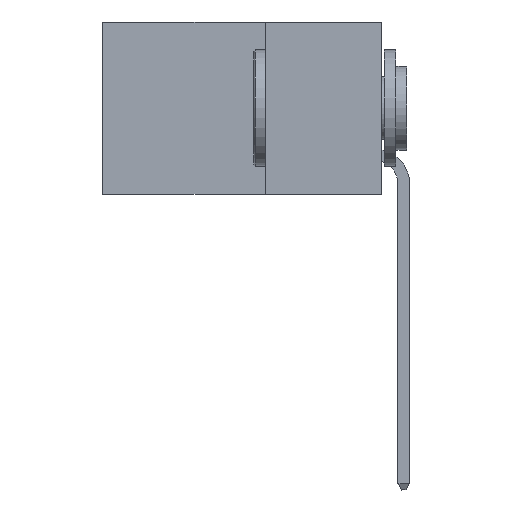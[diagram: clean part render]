
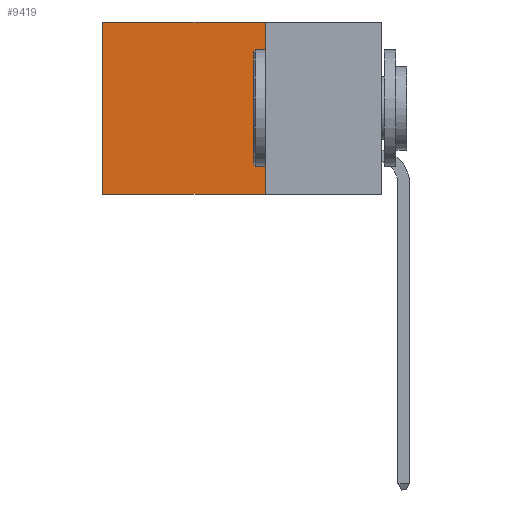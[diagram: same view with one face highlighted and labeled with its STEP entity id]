
A CAD part, left-side view. The second image highlights one B-rep face of the part: STEP entity #9419.
In plain terms, the highlighted planar face has unit normal (-1, 0, 0).
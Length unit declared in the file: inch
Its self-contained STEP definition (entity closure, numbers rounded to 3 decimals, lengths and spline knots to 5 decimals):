
#2 = EDGE_CURVE ( 'NONE', #17617, #24704, #14192, .T. ) ;
#827 = CARTESIAN_POINT ( 'NONE',  ( 0.2875, 0.25, -0.37 ) ) ;
#1540 = LINE ( 'NONE', #19312, #7014 ) ;
#1626 = DIRECTION ( 'NONE',  ( 0., 0., -1. ) ) ;
#1886 = CARTESIAN_POINT ( 'NONE',  ( 0.2875, 0.25, 0. ) ) ;
#3583 = DIRECTION ( 'NONE',  ( 0., 1., 0. ) ) ;
#4084 = DIRECTION ( 'NONE',  ( 0., 0., -1. ) ) ;
#4148 = ORIENTED_EDGE ( 'NONE', *, *, #23896, .F. ) ;
#5484 = VECTOR ( 'NONE', #1626, 39.37008 ) ;
#6017 = PLANE ( 'NONE',  #13813 ) ;
#6112 = DIRECTION ( 'NONE',  ( 0., 0., -1. ) ) ;
#6855 = VERTEX_POINT ( 'NONE', #827 ) ;
#6882 = EDGE_CURVE ( 'NONE', #24704, #18723, #8126, .T. ) ;
#7014 = VECTOR ( 'NONE', #3583, 39.37008 ) ;
#7795 = ORIENTED_EDGE ( 'NONE', *, *, #6882, .T. ) ;
#8126 = LINE ( 'NONE', #9735, #22111 ) ;
#9419 = ADVANCED_FACE ( 'NONE', ( #23034 ), #6017, .F. ) ;
#9735 = CARTESIAN_POINT ( 'NONE',  ( 0.2875, 0.6, 0. ) ) ;
#9984 = CARTESIAN_POINT ( 'NONE',  ( 0.2875, 0.25, 0. ) ) ;
#10827 = CARTESIAN_POINT ( 'NONE',  ( 0.2875, 0.25, 0. ) ) ;
#11217 = DIRECTION ( 'NONE',  ( 0., 1., 0. ) ) ;
#11560 = EDGE_CURVE ( 'NONE', #6855, #18723, #1540, .T. ) ;
#13813 = AXIS2_PLACEMENT_3D ( 'NONE', #10827, #15616, #6112 ) ;
#14192 = LINE ( 'NONE', #1886, #30434 ) ;
#15616 = DIRECTION ( 'NONE',  ( 1., 0., 0. ) ) ;
#17617 = VERTEX_POINT ( 'NONE', #9984 ) ;
#18708 = EDGE_LOOP ( 'NONE', ( #7795, #24937, #4148, #22323 ) ) ;
#18723 = VERTEX_POINT ( 'NONE', #29151 ) ;
#19312 = CARTESIAN_POINT ( 'NONE',  ( 0.2875, 0.25, -0.37 ) ) ;
#22111 = VECTOR ( 'NONE', #4084, 39.37008 ) ;
#22323 = ORIENTED_EDGE ( 'NONE', *, *, #2, .T. ) ;
#22884 = CARTESIAN_POINT ( 'NONE',  ( 0.2875, 0.6, 0. ) ) ;
#23034 = FACE_OUTER_BOUND ( 'NONE', #18708, .T. ) ;
#23178 = LINE ( 'NONE', #27541, #5484 ) ;
#23896 = EDGE_CURVE ( 'NONE', #17617, #6855, #23178, .T. ) ;
#24704 = VERTEX_POINT ( 'NONE', #22884 ) ;
#24937 = ORIENTED_EDGE ( 'NONE', *, *, #11560, .F. ) ;
#27541 = CARTESIAN_POINT ( 'NONE',  ( 0.2875, 0.25, 0. ) ) ;
#29151 = CARTESIAN_POINT ( 'NONE',  ( 0.2875, 0.6, -0.37 ) ) ;
#30434 = VECTOR ( 'NONE', #11217, 39.37008 ) ;
